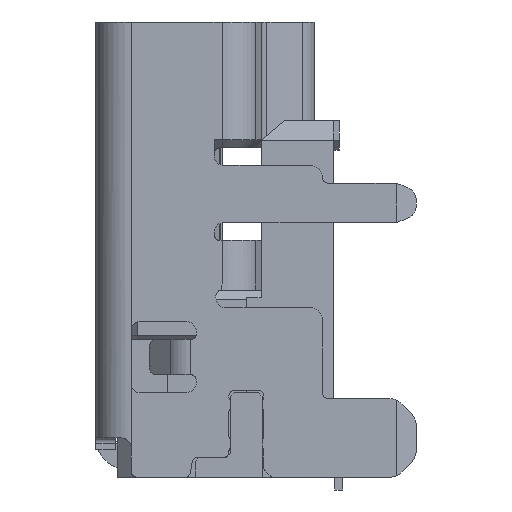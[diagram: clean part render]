
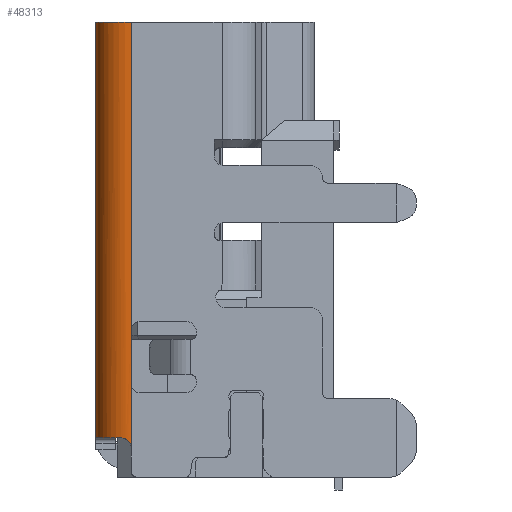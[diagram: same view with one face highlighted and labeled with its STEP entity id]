
A CAD part, left-side view. The second image highlights one B-rep face of the part: STEP entity #48313.
In plain terms, the highlighted cylindrical face has radius 0.9 mm (diameter 1.8 mm), a partial arc.
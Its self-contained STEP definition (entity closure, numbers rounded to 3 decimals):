
#681 = AXIS2_PLACEMENT_3D ( 'NONE', #17526, #24294, #3978 ) ;
#2446 = EDGE_CURVE ( 'NONE', #48249, #53514, #64070, .T. ) ;
#3978 = DIRECTION ( 'NONE',  ( 1., 0., 0. ) ) ;
#4588 = CARTESIAN_POINT ( 'NONE',  ( -7.501, -0.35, -8.171 ) ) ;
#5658 = DIRECTION ( 'NONE',  ( 1., 0., 0. ) ) ;
#7363 = EDGE_CURVE ( 'NONE', #53514, #45360, #62669, .T. ) ;
#7593 = EDGE_CURVE ( 'NONE', #45360, #13107, #18980, .T. ) ;
#8285 = CIRCLE ( 'NONE', #681, 0.9 ) ;
#9950 = EDGE_CURVE ( 'NONE', #37070, #48249, #22578, .T. ) ;
#12886 = EDGE_LOOP ( 'NONE', ( #27956, #16344, #56828, #46915, #13749, #22525, #38558 ) ) ;
#13107 = VERTEX_POINT ( 'NONE', #38341 ) ;
#13559 = DIRECTION ( 'NONE',  ( 0., 0., 1. ) ) ;
#13749 = ORIENTED_EDGE ( 'NONE', *, *, #59236, .T. ) ;
#16344 = ORIENTED_EDGE ( 'NONE', *, *, #7363, .T. ) ;
#17526 = CARTESIAN_POINT ( 'NONE',  ( -6.6, -0.375, 2.5 ) ) ;
#18980 = LINE ( 'NONE', #65007, #45087 ) ;
#20374 = DIRECTION ( 'NONE',  ( 0., 0., 1. ) ) ;
#20477 = CARTESIAN_POINT ( 'NONE',  ( -7.465, -0.125, -8.05 ) ) ;
#21133 = CARTESIAN_POINT ( 'NONE',  ( -7.5, -0.375, -8.23 ) ) ;
#21264 = EDGE_CURVE ( 'NONE', #53697, #37070, #49203, .T. ) ;
#22525 = ORIENTED_EDGE ( 'NONE', *, *, #21264, .T. ) ;
#22578 = CIRCLE ( 'NONE', #60370, 0.9 ) ;
#24294 = DIRECTION ( 'NONE',  ( 0., 0., -1. ) ) ;
#24950 = DIRECTION ( 'NONE',  ( 0., 0., 1. ) ) ;
#25240 = CARTESIAN_POINT ( 'NONE',  ( -7.5, -0.375, -8.3 ) ) ;
#27212 = CARTESIAN_POINT ( 'NONE',  ( -6.6, 0.525, -8.05 ) ) ;
#27956 = ORIENTED_EDGE ( 'NONE', *, *, #2446, .T. ) ;
#28569 = DIRECTION ( 'NONE',  ( 0., 0., -1. ) ) ;
#29706 = CYLINDRICAL_SURFACE ( 'NONE', #38369, 0.9 ) ;
#31419 = CARTESIAN_POINT ( 'NONE',  ( -6.6, -0.375, -8.05 ) ) ;
#31574 = CARTESIAN_POINT ( 'NONE',  ( -7.5, -0.375, 2.5 ) ) ;
#33807 = CARTESIAN_POINT ( 'NONE',  ( -7.465, -0.125, -8.05 ) ) ;
#36815 = CARTESIAN_POINT ( 'NONE',  ( -7.5, -0.375, 2.5 ) ) ;
#36953 = CARTESIAN_POINT ( 'NONE',  ( -7.5, -0.375, -8.3 ) ) ;
#37070 = VERTEX_POINT ( 'NONE', #27212 ) ;
#37610 = CARTESIAN_POINT ( 'NONE',  ( -7.5, -0.375, -6.7 ) ) ;
#37618 = CARTESIAN_POINT ( 'NONE',  ( -6.6, 0.525, 2.5 ) ) ;
#38341 = CARTESIAN_POINT ( 'NONE',  ( -7.5, -0.375, -5.3 ) ) ;
#38369 = AXIS2_PLACEMENT_3D ( 'NONE', #40204, #24950, #60479 ) ;
#38558 = ORIENTED_EDGE ( 'NONE', *, *, #9950, .T. ) ;
#39619 = VECTOR ( 'NONE', #20374, 1000. ) ;
#40204 = CARTESIAN_POINT ( 'NONE',  ( -6.6, -0.375, 2.5 ) ) ;
#43724 = CARTESIAN_POINT ( 'NONE',  ( -7.5, -0.375, 2.5 ) ) ;
#44712 = LINE ( 'NONE', #43724, #57164 ) ;
#45087 = VECTOR ( 'NONE', #13559, 1000. ) ;
#45360 = VERTEX_POINT ( 'NONE', #37610 ) ;
#46915 = ORIENTED_EDGE ( 'NONE', *, *, #52235, .T. ) ;
#48249 = VERTEX_POINT ( 'NONE', #33807 ) ;
#48313 = ADVANCED_FACE ( 'NONE', ( #55739 ), #29706, .T. ) ;
#48538 = VECTOR ( 'NONE', #28569, 1000. ) ;
#49203 = LINE ( 'NONE', #54946, #48538 ) ;
#52235 = EDGE_CURVE ( 'NONE', #13107, #60460, #44712, .T. ) ;
#53514 = VERTEX_POINT ( 'NONE', #36953 ) ;
#53697 = VERTEX_POINT ( 'NONE', #37618 ) ;
#54874 = DIRECTION ( 'NONE',  ( 0., 0., 1. ) ) ;
#54946 = CARTESIAN_POINT ( 'NONE',  ( -6.6, 0.525, 2.5 ) ) ;
#55739 = FACE_OUTER_BOUND ( 'NONE', #12886, .T. ) ;
#56828 = ORIENTED_EDGE ( 'NONE', *, *, #7593, .T. ) ;
#57164 = VECTOR ( 'NONE', #54874, 1000. ) ;
#58356 = DIRECTION ( 'NONE',  ( 0., 0., 1. ) ) ;
#59236 = EDGE_CURVE ( 'NONE', #60460, #53697, #8285, .T. ) ;
#60370 = AXIS2_PLACEMENT_3D ( 'NONE', #31419, #58356, #5658 ) ;
#60460 = VERTEX_POINT ( 'NONE', #36815 ) ;
#60479 = DIRECTION ( 'NONE',  ( 1., 0., 0. ) ) ;
#61081 = CARTESIAN_POINT ( 'NONE',  ( -7.493, -0.251, -8.073 ) ) ;
#62669 = LINE ( 'NONE', #31574, #39619 ) ;
#64070 = B_SPLINE_CURVE_WITH_KNOTS ( 'NONE', 3,
 ( #20477, #66823, #61081, #4588, #21133, #25240 ),
 .UNSPECIFIED., .F., .F.,
 ( 4, 2, 4 ),
 ( 0., 0.5, 1. ),
 .UNSPECIFIED. ) ;
#65007 = CARTESIAN_POINT ( 'NONE',  ( -7.5, -0.375, 2.5 ) ) ;
#66823 = CARTESIAN_POINT ( 'NONE',  ( -7.484, -0.193, -8.05 ) ) ;
